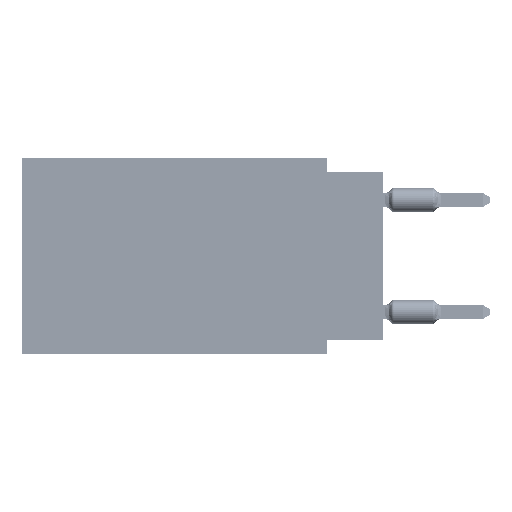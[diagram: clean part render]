
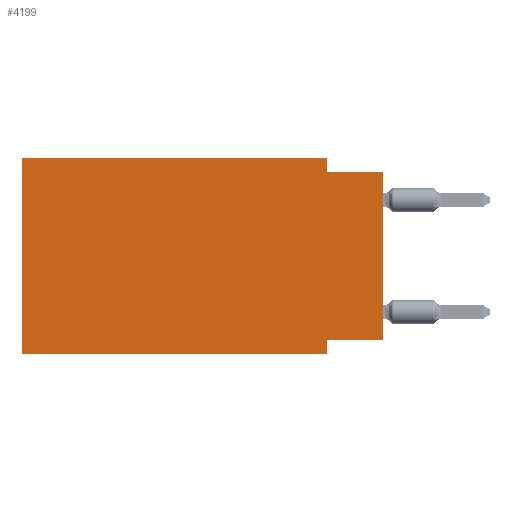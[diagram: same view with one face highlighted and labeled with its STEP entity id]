
A CAD part, left-side view. The second image highlights one B-rep face of the part: STEP entity #4199.
In plain terms, the highlighted planar face has unit normal (-1, 0, 0).
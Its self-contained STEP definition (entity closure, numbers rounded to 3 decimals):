
#74 = CARTESIAN_POINT ( 'NONE',  ( 0., 16.383, -8.89 ) ) ;
#1103 = LINE ( 'NONE', #21109, #10071 ) ;
#1350 = CARTESIAN_POINT ( 'NONE',  ( 0., 2.54, 0. ) ) ;
#2440 = EDGE_CURVE ( 'NONE', #16515, #62138, #22761, .T. ) ;
#2755 = VERTEX_POINT ( 'NONE', #51482 ) ;
#4153 = CARTESIAN_POINT ( 'NONE',  ( 0., 0., -8.255 ) ) ;
#4199 = ADVANCED_FACE ( 'NONE', ( #55428 ), #11450, .F. ) ;
#4289 = ORIENTED_EDGE ( 'NONE', *, *, #31098, .F. ) ;
#4418 = ORIENTED_EDGE ( 'NONE', *, *, #12880, .F. ) ;
#5020 = DIRECTION ( 'NONE',  ( 0., 0., -1. ) ) ;
#10071 = VECTOR ( 'NONE', #41132, 1000. ) ;
#11450 = PLANE ( 'NONE',  #49634 ) ;
#11802 = LINE ( 'NONE', #61341, #50492 ) ;
#12880 = EDGE_CURVE ( 'NONE', #52948, #34693, #47572, .T. ) ;
#12894 = VERTEX_POINT ( 'NONE', #33165 ) ;
#13854 = VERTEX_POINT ( 'NONE', #74 ) ;
#14266 = VECTOR ( 'NONE', #44542, 1000. ) ;
#14588 = ORIENTED_EDGE ( 'NONE', *, *, #2440, .T. ) ;
#15931 = ORIENTED_EDGE ( 'NONE', *, *, #50848, .F. ) ;
#16515 = VERTEX_POINT ( 'NONE', #4153 ) ;
#16741 = EDGE_CURVE ( 'NONE', #16515, #12894, #43136, .T. ) ;
#19797 = CARTESIAN_POINT ( 'NONE',  ( 0., 2.54, -8.89 ) ) ;
#21109 = CARTESIAN_POINT ( 'NONE',  ( 0., 0., -0.635 ) ) ;
#21298 = CARTESIAN_POINT ( 'NONE',  ( 0., 16.383, 0. ) ) ;
#21835 = DIRECTION ( 'NONE',  ( 0., 1., 0. ) ) ;
#22364 = VECTOR ( 'NONE', #5020, 1000. ) ;
#22761 = LINE ( 'NONE', #36897, #38010 ) ;
#22765 = VECTOR ( 'NONE', #51845, 1000. ) ;
#23231 = EDGE_CURVE ( 'NONE', #34693, #2755, #24543, .T. ) ;
#24009 = CARTESIAN_POINT ( 'NONE',  ( 0., 0., -0.635 ) ) ;
#24543 = LINE ( 'NONE', #61500, #14266 ) ;
#28066 = CARTESIAN_POINT ( 'NONE',  ( 0., 0., -8.255 ) ) ;
#31098 = EDGE_CURVE ( 'NONE', #13854, #52948, #11802, .T. ) ;
#31477 = DIRECTION ( 'NONE',  ( 0., 0., -1. ) ) ;
#31869 = CARTESIAN_POINT ( 'NONE',  ( 0., 16.383, 0. ) ) ;
#33165 = CARTESIAN_POINT ( 'NONE',  ( 0., 2.54, -8.255 ) ) ;
#34693 = VERTEX_POINT ( 'NONE', #1350 ) ;
#36895 = VECTOR ( 'NONE', #21835, 1000. ) ;
#36897 = CARTESIAN_POINT ( 'NONE',  ( 0., 0., 0. ) ) ;
#37714 = VECTOR ( 'NONE', #54838, 1000. ) ;
#38010 = VECTOR ( 'NONE', #46717, 1000. ) ;
#38806 = LINE ( 'NONE', #53879, #37714 ) ;
#39996 = VERTEX_POINT ( 'NONE', #53814 ) ;
#41132 = DIRECTION ( 'NONE',  ( 0., -1., 0. ) ) ;
#41320 = DIRECTION ( 'NONE',  ( 1., 0., 0. ) ) ;
#41379 = ORIENTED_EDGE ( 'NONE', *, *, #63038, .F. ) ;
#42845 = ORIENTED_EDGE ( 'NONE', *, *, #16741, .F. ) ;
#43136 = LINE ( 'NONE', #28066, #36895 ) ;
#43175 = EDGE_CURVE ( 'NONE', #13854, #39996, #38806, .T. ) ;
#44195 = ORIENTED_EDGE ( 'NONE', *, *, #23231, .F. ) ;
#44542 = DIRECTION ( 'NONE',  ( 0., 0., -1. ) ) ;
#46717 = DIRECTION ( 'NONE',  ( 0., 0., 1. ) ) ;
#47045 = EDGE_LOOP ( 'NONE', ( #14588, #41379, #44195, #4418, #4289, #62835, #15931, #42845 ) ) ;
#47572 = LINE ( 'NONE', #31869, #22765 ) ;
#49634 = AXIS2_PLACEMENT_3D ( 'NONE', #21298, #41320, #31477 ) ;
#50492 = VECTOR ( 'NONE', #61022, 1000. ) ;
#50848 = EDGE_CURVE ( 'NONE', #12894, #39996, #54888, .T. ) ;
#51482 = CARTESIAN_POINT ( 'NONE',  ( 0., 2.54, -0.635 ) ) ;
#51845 = DIRECTION ( 'NONE',  ( 0., -1., 0. ) ) ;
#52948 = VERTEX_POINT ( 'NONE', #56168 ) ;
#53814 = CARTESIAN_POINT ( 'NONE',  ( 0., 2.54, -8.89 ) ) ;
#53879 = CARTESIAN_POINT ( 'NONE',  ( 0., 16.383, -8.89 ) ) ;
#54838 = DIRECTION ( 'NONE',  ( 0., -1., 0. ) ) ;
#54888 = LINE ( 'NONE', #19797, #22364 ) ;
#55428 = FACE_OUTER_BOUND ( 'NONE', #47045, .T. ) ;
#56168 = CARTESIAN_POINT ( 'NONE',  ( 0., 16.383, 0. ) ) ;
#61022 = DIRECTION ( 'NONE',  ( 0., 0., 1. ) ) ;
#61341 = CARTESIAN_POINT ( 'NONE',  ( 0., 16.383, 0. ) ) ;
#61500 = CARTESIAN_POINT ( 'NONE',  ( 0., 2.54, 0. ) ) ;
#62138 = VERTEX_POINT ( 'NONE', #24009 ) ;
#62835 = ORIENTED_EDGE ( 'NONE', *, *, #43175, .T. ) ;
#63038 = EDGE_CURVE ( 'NONE', #2755, #62138, #1103, .T. ) ;
